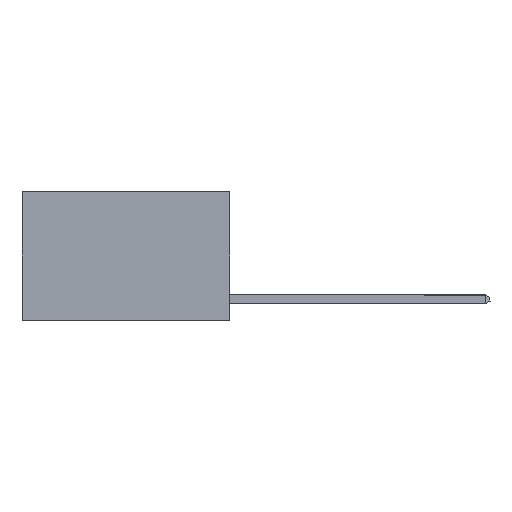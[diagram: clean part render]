
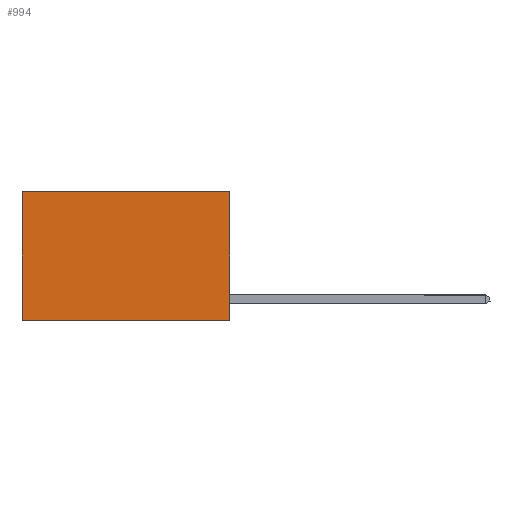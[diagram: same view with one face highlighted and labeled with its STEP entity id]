
A CAD part, left-side view. The second image highlights one B-rep face of the part: STEP entity #994.
In plain terms, the highlighted planar face has unit normal (-1, 0, 0).
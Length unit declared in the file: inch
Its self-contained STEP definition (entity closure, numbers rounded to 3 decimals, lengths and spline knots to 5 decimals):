
#299 = DIRECTION ( 'NONE',  ( 0., 1., 0. ) ) ;
#452 = DIRECTION ( 'NONE',  ( 0., 1., 0. ) ) ;
#994 = ADVANCED_FACE ( 'NONE', ( #15632 ), #13586, .F. ) ;
#1557 = ORIENTED_EDGE ( 'NONE', *, *, #9976, .T. ) ;
#3330 = EDGE_CURVE ( 'NONE', #6467, #10881, #11068, .T. ) ;
#3558 = VECTOR ( 'NONE', #299, 39.37008 ) ;
#3612 = CARTESIAN_POINT ( 'NONE',  ( 0.2625, 0.6, 0. ) ) ;
#3848 = VECTOR ( 'NONE', #452, 39.37008 ) ;
#4031 = VERTEX_POINT ( 'NONE', #4636 ) ;
#4636 = CARTESIAN_POINT ( 'NONE',  ( 0.2625, 0., 0. ) ) ;
#5968 = DIRECTION ( 'NONE',  ( 0., 0., -1. ) ) ;
#6467 = VERTEX_POINT ( 'NONE', #10619 ) ;
#6578 = DIRECTION ( 'NONE',  ( 0., 0., -1. ) ) ;
#7075 = CARTESIAN_POINT ( 'NONE',  ( 0.2625, 0., 0. ) ) ;
#7345 = CARTESIAN_POINT ( 'NONE',  ( 0.2625, 0.6, 0. ) ) ;
#7365 = EDGE_CURVE ( 'NONE', #4031, #12160, #11214, .T. ) ;
#7371 = VECTOR ( 'NONE', #6578, 39.37008 ) ;
#7733 = CARTESIAN_POINT ( 'NONE',  ( 0.2625, 0.6, -0.37 ) ) ;
#7795 = EDGE_LOOP ( 'NONE', ( #1557, #11602, #15678, #12632 ) ) ;
#8179 = VECTOR ( 'NONE', #5968, 39.37008 ) ;
#8335 = EDGE_CURVE ( 'NONE', #4031, #6467, #11376, .T. ) ;
#9976 = EDGE_CURVE ( 'NONE', #12160, #10881, #11727, .T. ) ;
#10619 = CARTESIAN_POINT ( 'NONE',  ( 0.2625, 0., -0.37 ) ) ;
#10881 = VERTEX_POINT ( 'NONE', #7733 ) ;
#11068 = LINE ( 'NONE', #11302, #3848 ) ;
#11214 = LINE ( 'NONE', #7075, #3558 ) ;
#11302 = CARTESIAN_POINT ( 'NONE',  ( 0.2625, 0., -0.37 ) ) ;
#11376 = LINE ( 'NONE', #15999, #7371 ) ;
#11602 = ORIENTED_EDGE ( 'NONE', *, *, #3330, .F. ) ;
#11727 = LINE ( 'NONE', #7345, #8179 ) ;
#12104 = AXIS2_PLACEMENT_3D ( 'NONE', #13702, #13546, #13462 ) ;
#12160 = VERTEX_POINT ( 'NONE', #3612 ) ;
#12632 = ORIENTED_EDGE ( 'NONE', *, *, #7365, .T. ) ;
#13462 = DIRECTION ( 'NONE',  ( 0., 0., -1. ) ) ;
#13546 = DIRECTION ( 'NONE',  ( 1., 0., 0. ) ) ;
#13586 = PLANE ( 'NONE',  #12104 ) ;
#13702 = CARTESIAN_POINT ( 'NONE',  ( 0.2625, 0., 0. ) ) ;
#15632 = FACE_OUTER_BOUND ( 'NONE', #7795, .T. ) ;
#15678 = ORIENTED_EDGE ( 'NONE', *, *, #8335, .F. ) ;
#15999 = CARTESIAN_POINT ( 'NONE',  ( 0.2625, 0., 0. ) ) ;
